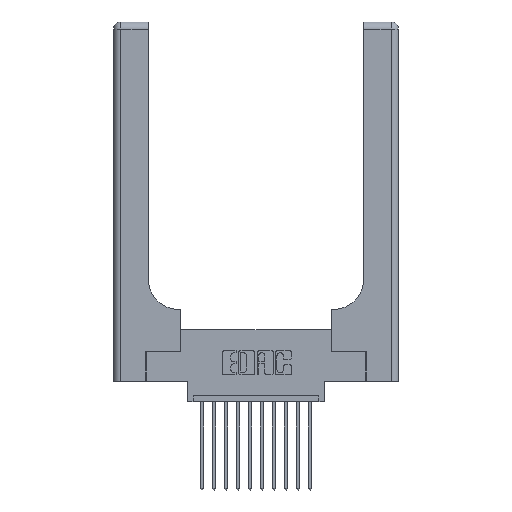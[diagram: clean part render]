
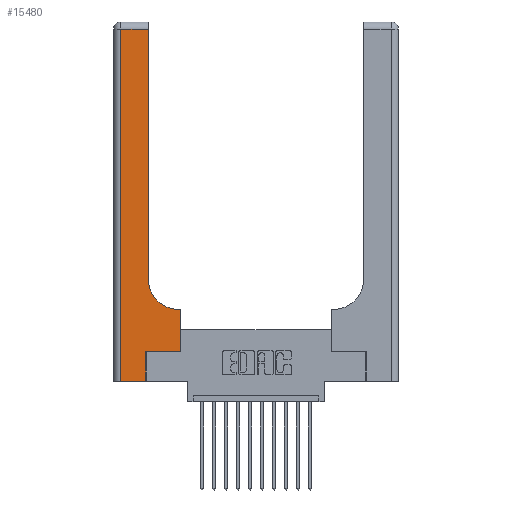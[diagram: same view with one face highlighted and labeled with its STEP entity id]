
A CAD part, top view. The second image highlights one B-rep face of the part: STEP entity #15480.
In plain terms, the highlighted planar face has unit normal (0, 0, 1).
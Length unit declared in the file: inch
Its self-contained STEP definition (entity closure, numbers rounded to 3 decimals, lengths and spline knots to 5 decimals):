
#269 = CARTESIAN_POINT ( 'NONE',  ( 0.269, 0., 0.37 ) ) ;
#333 = DIRECTION ( 'NONE',  ( 0., 1., 0. ) ) ;
#679 = VECTOR ( 'NONE', #2774, 39.37008 ) ;
#703 = CARTESIAN_POINT ( 'NONE',  ( 0.06, 3., 0.37 ) ) ;
#804 = ORIENTED_EDGE ( 'NONE', *, *, #12099, .T. ) ;
#1162 = VECTOR ( 'NONE', #12469, 39.37008 ) ;
#1167 = CARTESIAN_POINT ( 'NONE',  ( 0.2915, 3., 0.37 ) ) ;
#2228 = LINE ( 'NONE', #703, #5595 ) ;
#2229 = EDGE_CURVE ( 'NONE', #8455, #16958, #10851, .T. ) ;
#2419 = CARTESIAN_POINT ( 'NONE',  ( 0.2915, 0.6, 0.37 ) ) ;
#2774 = DIRECTION ( 'NONE',  ( 0., 1., 0. ) ) ;
#2999 = CARTESIAN_POINT ( 'NONE',  ( 0.5415, 0.85, 0.37 ) ) ;
#3119 = PLANE ( 'NONE',  #10038 ) ;
#3476 = LINE ( 'NONE', #2419, #8639 ) ;
#3942 = CARTESIAN_POINT ( 'NONE',  ( 0.269, 0., 0.37 ) ) ;
#4349 = LINE ( 'NONE', #269, #13013 ) ;
#4377 = DIRECTION ( 'NONE',  ( 0., 0., -1. ) ) ;
#4431 = DIRECTION ( 'NONE',  ( -1., 0., 0. ) ) ;
#4717 = CARTESIAN_POINT ( 'NONE',  ( 0.06, 0., 0.37 ) ) ;
#4835 = CARTESIAN_POINT ( 'NONE',  ( 0.2915, 0.85, 0.37 ) ) ;
#5008 = VERTEX_POINT ( 'NONE', #16912 ) ;
#5145 = LINE ( 'NONE', #15352, #1162 ) ;
#5407 = ORIENTED_EDGE ( 'NONE', *, *, #2229, .T. ) ;
#5518 = VERTEX_POINT ( 'NONE', #6037 ) ;
#5595 = VECTOR ( 'NONE', #12365, 39.37008 ) ;
#5697 = EDGE_CURVE ( 'NONE', #7553, #8169, #3476, .T. ) ;
#6037 = CARTESIAN_POINT ( 'NONE',  ( 0.2915, 2.94, 0.37 ) ) ;
#6510 = CARTESIAN_POINT ( 'NONE',  ( 0., 0., 0.37 ) ) ;
#6754 = CARTESIAN_POINT ( 'NONE',  ( 0.5585, 0.25, 0.37 ) ) ;
#7102 = ORIENTED_EDGE ( 'NONE', *, *, #16799, .T. ) ;
#7553 = VERTEX_POINT ( 'NONE', #16286 ) ;
#7832 = VERTEX_POINT ( 'NONE', #9449 ) ;
#7982 = VECTOR ( 'NONE', #15756, 39.37008 ) ;
#8169 = VERTEX_POINT ( 'NONE', #14952 ) ;
#8455 = VERTEX_POINT ( 'NONE', #4717 ) ;
#8639 = VECTOR ( 'NONE', #8791, 39.37008 ) ;
#8791 = DIRECTION ( 'NONE',  ( -1., 0., 0. ) ) ;
#8999 = LINE ( 'NONE', #6754, #679 ) ;
#9355 = VECTOR ( 'NONE', #11947, 39.37008 ) ;
#9449 = CARTESIAN_POINT ( 'NONE',  ( 0.5585, 0.25, 0.37 ) ) ;
#9918 = LINE ( 'NONE', #11161, #13856 ) ;
#9922 = CARTESIAN_POINT ( 'NONE',  ( 0.06, 2.94, 0.37 ) ) ;
#9949 = ORIENTED_EDGE ( 'NONE', *, *, #5697, .T. ) ;
#10038 = AXIS2_PLACEMENT_3D ( 'NONE', #10995, #12347, #4431 ) ;
#10324 = VERTEX_POINT ( 'NONE', #9922 ) ;
#10463 = ORIENTED_EDGE ( 'NONE', *, *, #16053, .T. ) ;
#10817 = ORIENTED_EDGE ( 'NONE', *, *, #16114, .T. ) ;
#10851 = LINE ( 'NONE', #6510, #7982 ) ;
#10995 = CARTESIAN_POINT ( 'NONE',  ( 0., 3., 0.37 ) ) ;
#11161 = CARTESIAN_POINT ( 'NONE',  ( 0., 2.94, 0.37 ) ) ;
#11274 = ORIENTED_EDGE ( 'NONE', *, *, #15447, .T. ) ;
#11947 = DIRECTION ( 'NONE',  ( 0., 1., 0. ) ) ;
#12099 = EDGE_CURVE ( 'NONE', #7832, #7553, #8999, .T. ) ;
#12139 = AXIS2_PLACEMENT_3D ( 'NONE', #2999, #4377, #12162 ) ;
#12162 = DIRECTION ( 'NONE',  ( 1., 0., 0. ) ) ;
#12347 = DIRECTION ( 'NONE',  ( 0., 0., -1. ) ) ;
#12365 = DIRECTION ( 'NONE',  ( 0., -1., 0. ) ) ;
#12453 = LINE ( 'NONE', #1167, #9355 ) ;
#12469 = DIRECTION ( 'NONE',  ( 1., 0., 0. ) ) ;
#12530 = ORIENTED_EDGE ( 'NONE', *, *, #15251, .T. ) ;
#12575 = DIRECTION ( 'NONE',  ( -1., 0., 0. ) ) ;
#13013 = VECTOR ( 'NONE', #333, 39.37008 ) ;
#13856 = VECTOR ( 'NONE', #12575, 39.37008 ) ;
#13905 = VERTEX_POINT ( 'NONE', #4835 ) ;
#14645 = EDGE_CURVE ( 'NONE', #13905, #5518, #12453, .T. ) ;
#14713 = CIRCLE ( 'NONE', #12139, 0.25 ) ;
#14952 = CARTESIAN_POINT ( 'NONE',  ( 0.5415, 0.6, 0.37 ) ) ;
#15251 = EDGE_CURVE ( 'NONE', #8169, #13905, #14713, .T. ) ;
#15336 = EDGE_LOOP ( 'NONE', ( #17089, #11274, #10817, #5407, #10463, #7102, #804, #9949, #12530 ) ) ;
#15352 = CARTESIAN_POINT ( 'NONE',  ( 0.269, 0.25, 0.37 ) ) ;
#15447 = EDGE_CURVE ( 'NONE', #5518, #10324, #9918, .T. ) ;
#15480 = ADVANCED_FACE ( 'NONE', ( #16547 ), #3119, .F. ) ;
#15756 = DIRECTION ( 'NONE',  ( 1., 0., 0. ) ) ;
#16053 = EDGE_CURVE ( 'NONE', #16958, #5008, #4349, .T. ) ;
#16114 = EDGE_CURVE ( 'NONE', #10324, #8455, #2228, .T. ) ;
#16286 = CARTESIAN_POINT ( 'NONE',  ( 0.5585, 0.6, 0.37 ) ) ;
#16547 = FACE_OUTER_BOUND ( 'NONE', #15336, .T. ) ;
#16799 = EDGE_CURVE ( 'NONE', #5008, #7832, #5145, .T. ) ;
#16912 = CARTESIAN_POINT ( 'NONE',  ( 0.269, 0.25, 0.37 ) ) ;
#16958 = VERTEX_POINT ( 'NONE', #3942 ) ;
#17089 = ORIENTED_EDGE ( 'NONE', *, *, #14645, .T. ) ;
